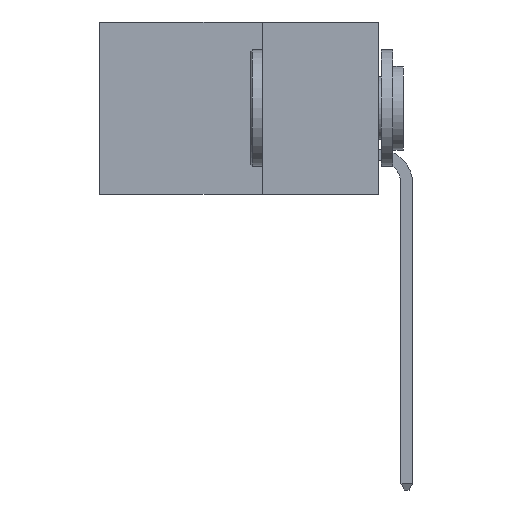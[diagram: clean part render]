
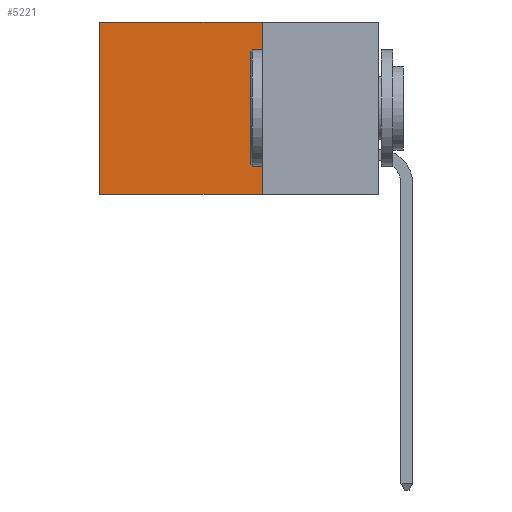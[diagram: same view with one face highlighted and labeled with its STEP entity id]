
A CAD part, left-side view. The second image highlights one B-rep face of the part: STEP entity #5221.
In plain terms, the highlighted planar face has unit normal (-1, 0, 0).
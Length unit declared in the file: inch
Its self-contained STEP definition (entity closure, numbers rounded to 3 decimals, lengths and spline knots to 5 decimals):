
#311 = CARTESIAN_POINT ( 'NONE',  ( 0.2615, 0.6, 0. ) ) ;
#705 = EDGE_CURVE ( 'NONE', #9011, #6111, #2392, .T. ) ;
#1447 = CARTESIAN_POINT ( 'NONE',  ( 0.2615, 0.25, -0.37 ) ) ;
#1747 = EDGE_CURVE ( 'NONE', #9289, #4281, #4869, .T. ) ;
#2159 = VECTOR ( 'NONE', #11353, 39.37008 ) ;
#2392 = LINE ( 'NONE', #1447, #2721 ) ;
#2519 = EDGE_CURVE ( 'NONE', #6111, #4281, #5163, .T. ) ;
#2721 = VECTOR ( 'NONE', #5554, 39.37008 ) ;
#3732 = CARTESIAN_POINT ( 'NONE',  ( 0.2615, 0.6, -0.37 ) ) ;
#3912 = PLANE ( 'NONE',  #7974 ) ;
#4092 = CARTESIAN_POINT ( 'NONE',  ( 0.2615, 0.25, 0. ) ) ;
#4281 = VERTEX_POINT ( 'NONE', #3732 ) ;
#4485 = CARTESIAN_POINT ( 'NONE',  ( 0.2615, 0.25, 0. ) ) ;
#4869 = LINE ( 'NONE', #6447, #12300 ) ;
#4910 = DIRECTION ( 'NONE',  ( 1., 0., 0. ) ) ;
#5163 = LINE ( 'NONE', #11674, #12573 ) ;
#5221 = ADVANCED_FACE ( 'NONE', ( #6343 ), #3912, .F. ) ;
#5554 = DIRECTION ( 'NONE',  ( 0., 0., -1. ) ) ;
#6111 = VERTEX_POINT ( 'NONE', #11977 ) ;
#6343 = FACE_OUTER_BOUND ( 'NONE', #9844, .T. ) ;
#6437 = DIRECTION ( 'NONE',  ( 0., 0., -1. ) ) ;
#6447 = CARTESIAN_POINT ( 'NONE',  ( 0.2615, 0.6, -0.37 ) ) ;
#7495 = LINE ( 'NONE', #4485, #2159 ) ;
#7536 = ORIENTED_EDGE ( 'NONE', *, *, #705, .F. ) ;
#7974 = AXIS2_PLACEMENT_3D ( 'NONE', #10730, #4910, #11715 ) ;
#7983 = EDGE_CURVE ( 'NONE', #9011, #9289, #7495, .T. ) ;
#8595 = DIRECTION ( 'NONE',  ( 0., 1., 0. ) ) ;
#9011 = VERTEX_POINT ( 'NONE', #4092 ) ;
#9289 = VERTEX_POINT ( 'NONE', #311 ) ;
#9844 = EDGE_LOOP ( 'NONE', ( #12629, #11900, #7536, #10853 ) ) ;
#10730 = CARTESIAN_POINT ( 'NONE',  ( 0.2615, 0.25, -0.37 ) ) ;
#10853 = ORIENTED_EDGE ( 'NONE', *, *, #7983, .T. ) ;
#11353 = DIRECTION ( 'NONE',  ( 0., 1., 0. ) ) ;
#11674 = CARTESIAN_POINT ( 'NONE',  ( 0.2615, 0.25, -0.37 ) ) ;
#11715 = DIRECTION ( 'NONE',  ( 0., 0., -1. ) ) ;
#11900 = ORIENTED_EDGE ( 'NONE', *, *, #2519, .F. ) ;
#11977 = CARTESIAN_POINT ( 'NONE',  ( 0.2615, 0.25, -0.37 ) ) ;
#12300 = VECTOR ( 'NONE', #6437, 39.37008 ) ;
#12573 = VECTOR ( 'NONE', #8595, 39.37008 ) ;
#12629 = ORIENTED_EDGE ( 'NONE', *, *, #1747, .T. ) ;
